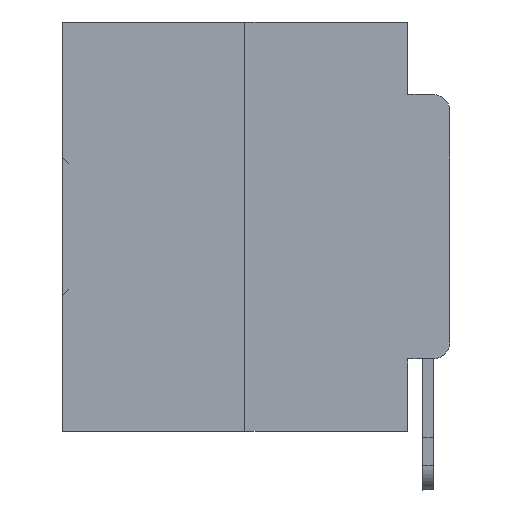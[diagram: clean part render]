
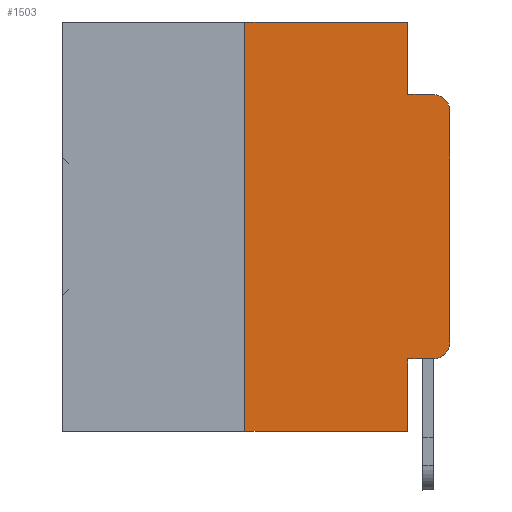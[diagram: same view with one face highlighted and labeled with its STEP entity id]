
A CAD part, left-side view. The second image highlights one B-rep face of the part: STEP entity #1503.
In plain terms, the highlighted planar face has unit normal (-1, 0, 0).
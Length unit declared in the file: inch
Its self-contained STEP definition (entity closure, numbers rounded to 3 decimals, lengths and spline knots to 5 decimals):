
#122 = CARTESIAN_POINT ( 'NONE',  ( 0., 0.051, 0. ) ) ;
#464 = VECTOR ( 'NONE', #16355, 39.37008 ) ;
#1134 = VECTOR ( 'NONE', #21472, 39.37008 ) ;
#1170 = CARTESIAN_POINT ( 'NONE',  ( 0., 0.051, -0.5 ) ) ;
#1503 = ADVANCED_FACE ( 'NONE', ( #20234 ), #13529, .F. ) ;
#2078 = LINE ( 'NONE', #16608, #30994 ) ;
#2431 = EDGE_CURVE ( 'NONE', #21148, #17289, #20569, .T. ) ;
#2720 = DIRECTION ( 'NONE',  ( 0., 0., -1. ) ) ;
#3506 = AXIS2_PLACEMENT_3D ( 'NONE', #13764, #21709, #21928 ) ;
#4354 = CARTESIAN_POINT ( 'NONE',  ( 0., 0.02, -0.0885 ) ) ;
#4705 = CARTESIAN_POINT ( 'NONE',  ( 0., 0.051, 0. ) ) ;
#5206 = CARTESIAN_POINT ( 'NONE',  ( 0., 0.02, -0.4115 ) ) ;
#5311 = DIRECTION ( 'NONE',  ( -1., 0., 0. ) ) ;
#6033 = ORIENTED_EDGE ( 'NONE', *, *, #31230, .T. ) ;
#6161 = CARTESIAN_POINT ( 'NONE',  ( 0., 0., -0.3915 ) ) ;
#6408 = VECTOR ( 'NONE', #10860, 39.37008 ) ;
#7017 = LINE ( 'NONE', #34532, #33872 ) ;
#7185 = ORIENTED_EDGE ( 'NONE', *, *, #24804, .F. ) ;
#7429 = ORIENTED_EDGE ( 'NONE', *, *, #17279, .F. ) ;
#9911 = CARTESIAN_POINT ( 'NONE',  ( 0., 0.051, -0.0885 ) ) ;
#10624 = CARTESIAN_POINT ( 'NONE',  ( 0., 0.051, -0.4115 ) ) ;
#10860 = DIRECTION ( 'NONE',  ( 0., -1., 0. ) ) ;
#11514 = EDGE_CURVE ( 'NONE', #34492, #18491, #17827, .T. ) ;
#11554 = VERTEX_POINT ( 'NONE', #9911 ) ;
#12124 = LINE ( 'NONE', #122, #27635 ) ;
#12574 = VERTEX_POINT ( 'NONE', #18451 ) ;
#12600 = CARTESIAN_POINT ( 'NONE',  ( 0., 0.02, -0.3915 ) ) ;
#12714 = DIRECTION ( 'NONE',  ( -1., 0., 0. ) ) ;
#13150 = ORIENTED_EDGE ( 'NONE', *, *, #32196, .F. ) ;
#13529 = PLANE ( 'NONE',  #3506 ) ;
#13764 = CARTESIAN_POINT ( 'NONE',  ( 0., 0.473, 0. ) ) ;
#14273 = CARTESIAN_POINT ( 'NONE',  ( 0., 0.25, -0.5 ) ) ;
#15173 = DIRECTION ( 'NONE',  ( 0., 0., -1. ) ) ;
#16266 = VERTEX_POINT ( 'NONE', #1170 ) ;
#16355 = DIRECTION ( 'NONE',  ( 0., -1., 0. ) ) ;
#16608 = CARTESIAN_POINT ( 'NONE',  ( 0., 0.473, -0.5 ) ) ;
#16729 = ORIENTED_EDGE ( 'NONE', *, *, #21596, .T. ) ;
#16870 = LINE ( 'NONE', #33902, #31925 ) ;
#17279 = EDGE_CURVE ( 'NONE', #17289, #32214, #25204, .T. ) ;
#17289 = VERTEX_POINT ( 'NONE', #24398 ) ;
#17685 = VERTEX_POINT ( 'NONE', #4354 ) ;
#17714 = AXIS2_PLACEMENT_3D ( 'NONE', #12600, #12714, #20700 ) ;
#17827 = CIRCLE ( 'NONE', #17714, 0.02 ) ;
#18451 = CARTESIAN_POINT ( 'NONE',  ( 0., 0.051, -0.4115 ) ) ;
#18491 = VERTEX_POINT ( 'NONE', #6161 ) ;
#18693 = CARTESIAN_POINT ( 'NONE',  ( 0., 0.02, -0.1085 ) ) ;
#18937 = CARTESIAN_POINT ( 'NONE',  ( 0., 0.25, 0. ) ) ;
#19618 = CARTESIAN_POINT ( 'NONE',  ( 0., 0., -0.1085 ) ) ;
#19871 = ORIENTED_EDGE ( 'NONE', *, *, #33604, .T. ) ;
#20234 = FACE_OUTER_BOUND ( 'NONE', #23285, .T. ) ;
#20569 = LINE ( 'NONE', #18937, #23889 ) ;
#20700 = DIRECTION ( 'NONE',  ( 0., 0., -1. ) ) ;
#21148 = VERTEX_POINT ( 'NONE', #14273 ) ;
#21253 = CARTESIAN_POINT ( 'NONE',  ( 0., 0.473, 0. ) ) ;
#21472 = DIRECTION ( 'NONE',  ( 0., -1., 0. ) ) ;
#21596 = EDGE_CURVE ( 'NONE', #29001, #17685, #21966, .T. ) ;
#21709 = DIRECTION ( 'NONE',  ( 1., 0., 0. ) ) ;
#21928 = DIRECTION ( 'NONE',  ( 0., 0., -1. ) ) ;
#21966 = CIRCLE ( 'NONE', #26149, 0.02 ) ;
#22509 = LINE ( 'NONE', #24277, #1134 ) ;
#23285 = EDGE_LOOP ( 'NONE', ( #25427, #16729, #7185, #13150, #7429, #27581, #19871, #26307, #6033, #30205 ) ) ;
#23889 = VECTOR ( 'NONE', #27449, 39.37008 ) ;
#23999 = DIRECTION ( 'NONE',  ( 0., 0., -1. ) ) ;
#24277 = CARTESIAN_POINT ( 'NONE',  ( 0., 0.051, -0.0885 ) ) ;
#24398 = CARTESIAN_POINT ( 'NONE',  ( 0., 0.25, 0. ) ) ;
#24804 = EDGE_CURVE ( 'NONE', #11554, #17685, #22509, .T. ) ;
#25204 = LINE ( 'NONE', #21253, #464 ) ;
#25427 = ORIENTED_EDGE ( 'NONE', *, *, #34465, .T. ) ;
#26149 = AXIS2_PLACEMENT_3D ( 'NONE', #18693, #5311, #2720 ) ;
#26307 = ORIENTED_EDGE ( 'NONE', *, *, #27682, .F. ) ;
#27123 = DIRECTION ( 'NONE',  ( 0., -1., 0. ) ) ;
#27449 = DIRECTION ( 'NONE',  ( 0., 0., 1. ) ) ;
#27581 = ORIENTED_EDGE ( 'NONE', *, *, #2431, .F. ) ;
#27635 = VECTOR ( 'NONE', #23999, 39.37008 ) ;
#27682 = EDGE_CURVE ( 'NONE', #12574, #16266, #12124, .T. ) ;
#27801 = LINE ( 'NONE', #10624, #6408 ) ;
#29001 = VERTEX_POINT ( 'NONE', #19618 ) ;
#30205 = ORIENTED_EDGE ( 'NONE', *, *, #11514, .T. ) ;
#30994 = VECTOR ( 'NONE', #27123, 39.37008 ) ;
#31230 = EDGE_CURVE ( 'NONE', #12574, #34492, #27801, .T. ) ;
#31925 = VECTOR ( 'NONE', #15173, 39.37008 ) ;
#32196 = EDGE_CURVE ( 'NONE', #32214, #11554, #16870, .T. ) ;
#32214 = VERTEX_POINT ( 'NONE', #4705 ) ;
#33604 = EDGE_CURVE ( 'NONE', #21148, #16266, #2078, .T. ) ;
#33872 = VECTOR ( 'NONE', #34419, 39.37008 ) ;
#33902 = CARTESIAN_POINT ( 'NONE',  ( 0., 0.051, 0. ) ) ;
#34419 = DIRECTION ( 'NONE',  ( 0., 0., 1. ) ) ;
#34465 = EDGE_CURVE ( 'NONE', #18491, #29001, #7017, .T. ) ;
#34492 = VERTEX_POINT ( 'NONE', #5206 ) ;
#34532 = CARTESIAN_POINT ( 'NONE',  ( 0., 0., 0. ) ) ;
